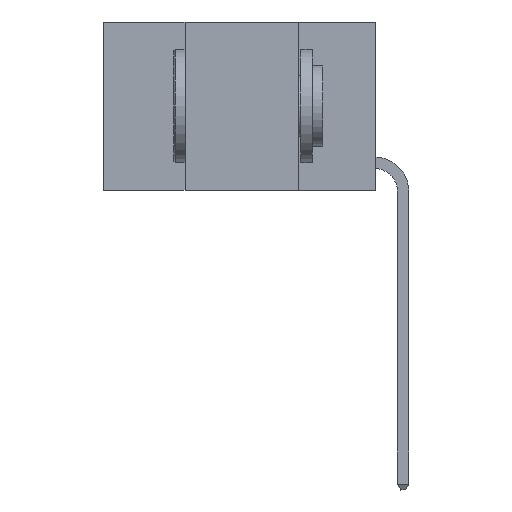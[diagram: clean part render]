
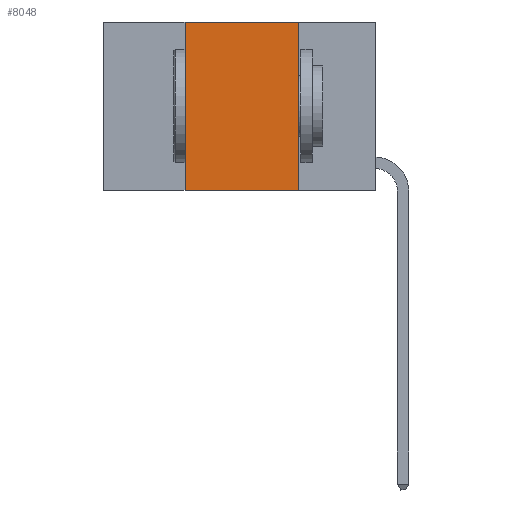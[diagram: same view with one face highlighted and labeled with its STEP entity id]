
A CAD part, left-side view. The second image highlights one B-rep face of the part: STEP entity #8048.
In plain terms, the highlighted planar face has unit normal (-1, 0, 0).
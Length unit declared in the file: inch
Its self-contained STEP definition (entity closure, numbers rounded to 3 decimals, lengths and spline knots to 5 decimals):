
#366 = DIRECTION ( 'NONE',  ( 0., 0., -1. ) ) ;
#398 = DIRECTION ( 'NONE',  ( 0., 0., -1. ) ) ;
#1197 = CARTESIAN_POINT ( 'NONE',  ( 0., 0.42, 0. ) ) ;
#1467 = LINE ( 'NONE', #20065, #3072 ) ;
#1588 = VERTEX_POINT ( 'NONE', #15346 ) ;
#2068 = CARTESIAN_POINT ( 'NONE',  ( 0., 0.42, 0. ) ) ;
#2295 = LINE ( 'NONE', #13203, #7892 ) ;
#2936 = CARTESIAN_POINT ( 'NONE',  ( 0., 0.6, 0. ) ) ;
#3065 = VERTEX_POINT ( 'NONE', #3576 ) ;
#3072 = VECTOR ( 'NONE', #15369, 39.37008 ) ;
#3576 = CARTESIAN_POINT ( 'NONE',  ( 0., 0.42, -0.37 ) ) ;
#3608 = LINE ( 'NONE', #2068, #9563 ) ;
#4675 = FACE_OUTER_BOUND ( 'NONE', #8301, .T. ) ;
#5522 = EDGE_CURVE ( 'NONE', #3065, #1588, #1467, .T. ) ;
#6404 = ORIENTED_EDGE ( 'NONE', *, *, #5522, .T. ) ;
#6683 = DIRECTION ( 'NONE',  ( 0., 0., 1. ) ) ;
#7892 = VECTOR ( 'NONE', #366, 39.37008 ) ;
#8048 = ADVANCED_FACE ( 'NONE', ( #4675 ), #8053, .F. ) ;
#8053 = PLANE ( 'NONE',  #13121 ) ;
#8301 = EDGE_LOOP ( 'NONE', ( #17661, #18793, #15281, #6404 ) ) ;
#8724 = EDGE_CURVE ( 'NONE', #11583, #1588, #2295, .T. ) ;
#9563 = VECTOR ( 'NONE', #6683, 39.37008 ) ;
#10145 = EDGE_CURVE ( 'NONE', #3065, #15820, #3608, .T. ) ;
#11135 = CARTESIAN_POINT ( 'NONE',  ( 0., 0.17, 0. ) ) ;
#11583 = VERTEX_POINT ( 'NONE', #11135 ) ;
#13121 = AXIS2_PLACEMENT_3D ( 'NONE', #15422, #18889, #398 ) ;
#13203 = CARTESIAN_POINT ( 'NONE',  ( 0., 0.17, 0. ) ) ;
#15281 = ORIENTED_EDGE ( 'NONE', *, *, #10145, .F. ) ;
#15346 = CARTESIAN_POINT ( 'NONE',  ( 0., 0.17, -0.37 ) ) ;
#15369 = DIRECTION ( 'NONE',  ( 0., -1., 0. ) ) ;
#15422 = CARTESIAN_POINT ( 'NONE',  ( 0., 0.6, 0. ) ) ;
#15428 = EDGE_CURVE ( 'NONE', #15820, #11583, #18294, .T. ) ;
#15820 = VERTEX_POINT ( 'NONE', #1197 ) ;
#17661 = ORIENTED_EDGE ( 'NONE', *, *, #8724, .F. ) ;
#18294 = LINE ( 'NONE', #2936, #18883 ) ;
#18793 = ORIENTED_EDGE ( 'NONE', *, *, #15428, .F. ) ;
#18883 = VECTOR ( 'NONE', #19713, 39.37008 ) ;
#18889 = DIRECTION ( 'NONE',  ( 1., 0., 0. ) ) ;
#19713 = DIRECTION ( 'NONE',  ( 0., -1., 0. ) ) ;
#20065 = CARTESIAN_POINT ( 'NONE',  ( 0., 0.6, -0.37 ) ) ;
